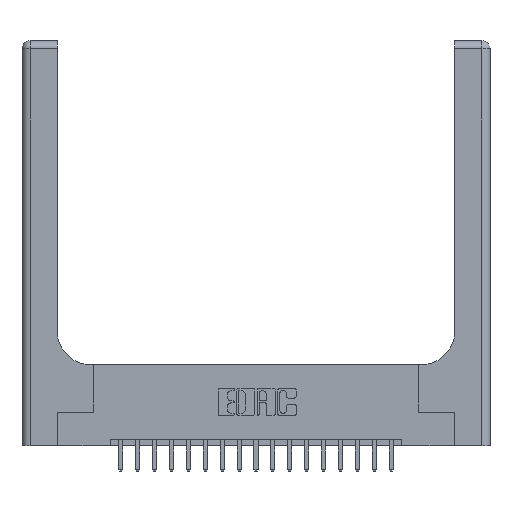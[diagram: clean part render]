
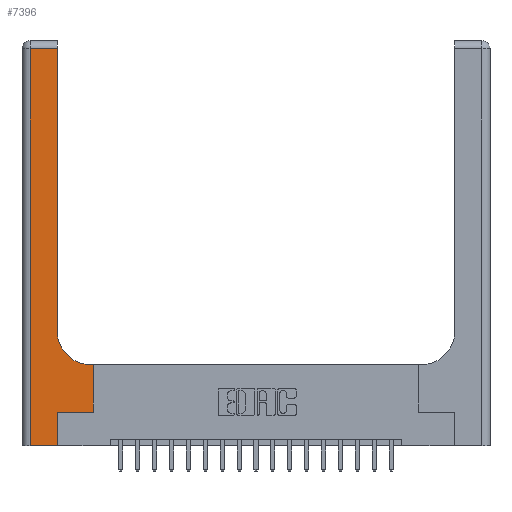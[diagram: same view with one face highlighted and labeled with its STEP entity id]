
A CAD part, top view. The second image highlights one B-rep face of the part: STEP entity #7396.
In plain terms, the highlighted planar face has unit normal (0, 0, 1).
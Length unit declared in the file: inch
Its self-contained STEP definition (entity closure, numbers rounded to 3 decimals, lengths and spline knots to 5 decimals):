
#52 = CARTESIAN_POINT ( 'NONE',  ( 0.26, 0.6, 0.37 ) ) ;
#112 = LINE ( 'NONE', #11116, #958 ) ;
#550 = CARTESIAN_POINT ( 'NONE',  ( 0.265, 0., 0.37 ) ) ;
#718 = CARTESIAN_POINT ( 'NONE',  ( 0.26, 2.94, 0.37 ) ) ;
#727 = CARTESIAN_POINT ( 'NONE',  ( 0., 0., 0.37 ) ) ;
#887 = ORIENTED_EDGE ( 'NONE', *, *, #5581, .T. ) ;
#958 = VECTOR ( 'NONE', #15806, 39.37008 ) ;
#1200 = LINE ( 'NONE', #727, #9588 ) ;
#1268 = EDGE_CURVE ( 'NONE', #19633, #1485, #16628, .T. ) ;
#1485 = VERTEX_POINT ( 'NONE', #2254 ) ;
#1619 = DIRECTION ( 'NONE',  ( -1., 0., 0. ) ) ;
#1894 = LINE ( 'NONE', #550, #2456 ) ;
#2235 = ORIENTED_EDGE ( 'NONE', *, *, #10881, .T. ) ;
#2254 = CARTESIAN_POINT ( 'NONE',  ( 0.06, 0., 0.37 ) ) ;
#2456 = VECTOR ( 'NONE', #17449, 39.37008 ) ;
#3403 = CARTESIAN_POINT ( 'NONE',  ( 0.265, 0.25, 0.37 ) ) ;
#3526 = VERTEX_POINT ( 'NONE', #4271 ) ;
#3614 = EDGE_CURVE ( 'NONE', #3526, #9872, #14115, .T. ) ;
#4226 = LINE ( 'NONE', #13772, #12684 ) ;
#4271 = CARTESIAN_POINT ( 'NONE',  ( 0.528, 0.6, 0.37 ) ) ;
#4289 = CARTESIAN_POINT ( 'NONE',  ( 0.06, 2.94, 0.37 ) ) ;
#4811 = AXIS2_PLACEMENT_3D ( 'NONE', #14265, #14073, #17016 ) ;
#5474 = DIRECTION ( 'NONE',  ( 0., -1., 0. ) ) ;
#5581 = EDGE_CURVE ( 'NONE', #6581, #9109, #112, .T. ) ;
#5914 = PLANE ( 'NONE',  #20081 ) ;
#5966 = DIRECTION ( 'NONE',  ( 1., 0., 0. ) ) ;
#6322 = DIRECTION ( 'NONE',  ( -1., 0., 0. ) ) ;
#6462 = ORIENTED_EDGE ( 'NONE', *, *, #18811, .T. ) ;
#6581 = VERTEX_POINT ( 'NONE', #7787 ) ;
#6842 = LINE ( 'NONE', #7458, #16123 ) ;
#7328 = ORIENTED_EDGE ( 'NONE', *, *, #3614, .T. ) ;
#7396 = ADVANCED_FACE ( 'NONE', ( #17382 ), #5914, .F. ) ;
#7412 = ORIENTED_EDGE ( 'NONE', *, *, #16473, .T. ) ;
#7458 = CARTESIAN_POINT ( 'NONE',  ( 0.265, 0.25, 0.37 ) ) ;
#7520 = ORIENTED_EDGE ( 'NONE', *, *, #16606, .T. ) ;
#7787 = CARTESIAN_POINT ( 'NONE',  ( 0.26, 0.85, 0.37 ) ) ;
#7793 = EDGE_CURVE ( 'NONE', #9057, #3526, #8575, .T. ) ;
#7808 = CARTESIAN_POINT ( 'NONE',  ( 0.51, 0.6, 0.37 ) ) ;
#8575 = LINE ( 'NONE', #11718, #14574 ) ;
#9057 = VERTEX_POINT ( 'NONE', #17623 ) ;
#9109 = VERTEX_POINT ( 'NONE', #718 ) ;
#9375 = CARTESIAN_POINT ( 'NONE',  ( 0.265, 0., 0.37 ) ) ;
#9588 = VECTOR ( 'NONE', #5966, 39.37008 ) ;
#9872 = VERTEX_POINT ( 'NONE', #7808 ) ;
#10029 = VECTOR ( 'NONE', #5474, 39.37008 ) ;
#10498 = DIRECTION ( 'NONE',  ( 0., 1., 0. ) ) ;
#10881 = EDGE_CURVE ( 'NONE', #1485, #17893, #1200, .T. ) ;
#11116 = CARTESIAN_POINT ( 'NONE',  ( 0.26, 3., 0.37 ) ) ;
#11326 = ORIENTED_EDGE ( 'NONE', *, *, #1268, .T. ) ;
#11406 = EDGE_LOOP ( 'NONE', ( #887, #7412, #11326, #2235, #6462, #12799, #16649, #7328, #7520 ) ) ;
#11561 = EDGE_CURVE ( 'NONE', #19064, #9057, #6842, .T. ) ;
#11718 = CARTESIAN_POINT ( 'NONE',  ( 0.528, 0.25, 0.37 ) ) ;
#12050 = DIRECTION ( 'NONE',  ( 1., 0., 0. ) ) ;
#12684 = VECTOR ( 'NONE', #16711, 39.37008 ) ;
#12799 = ORIENTED_EDGE ( 'NONE', *, *, #11561, .T. ) ;
#13772 = CARTESIAN_POINT ( 'NONE',  ( 0., 2.94, 0.37 ) ) ;
#13783 = DIRECTION ( 'NONE',  ( 0., 0., -1. ) ) ;
#14073 = DIRECTION ( 'NONE',  ( 0., 0., -1. ) ) ;
#14115 = LINE ( 'NONE', #52, #18869 ) ;
#14265 = CARTESIAN_POINT ( 'NONE',  ( 0.51, 0.85, 0.37 ) ) ;
#14574 = VECTOR ( 'NONE', #10498, 39.37008 ) ;
#15806 = DIRECTION ( 'NONE',  ( 0., 1., 0. ) ) ;
#16123 = VECTOR ( 'NONE', #12050, 39.37008 ) ;
#16473 = EDGE_CURVE ( 'NONE', #9109, #19633, #4226, .T. ) ;
#16606 = EDGE_CURVE ( 'NONE', #9872, #6581, #17527, .T. ) ;
#16628 = LINE ( 'NONE', #19457, #10029 ) ;
#16649 = ORIENTED_EDGE ( 'NONE', *, *, #7793, .T. ) ;
#16711 = DIRECTION ( 'NONE',  ( -1., 0., 0. ) ) ;
#17016 = DIRECTION ( 'NONE',  ( 1., 0., 0. ) ) ;
#17382 = FACE_OUTER_BOUND ( 'NONE', #11406, .T. ) ;
#17449 = DIRECTION ( 'NONE',  ( 0., 1., 0. ) ) ;
#17527 = CIRCLE ( 'NONE', #4811, 0.25 ) ;
#17623 = CARTESIAN_POINT ( 'NONE',  ( 0.528, 0.25, 0.37 ) ) ;
#17893 = VERTEX_POINT ( 'NONE', #9375 ) ;
#18811 = EDGE_CURVE ( 'NONE', #17893, #19064, #1894, .T. ) ;
#18818 = CARTESIAN_POINT ( 'NONE',  ( 0., 3., 0.37 ) ) ;
#18869 = VECTOR ( 'NONE', #6322, 39.37008 ) ;
#19064 = VERTEX_POINT ( 'NONE', #3403 ) ;
#19457 = CARTESIAN_POINT ( 'NONE',  ( 0.06, 3., 0.37 ) ) ;
#19633 = VERTEX_POINT ( 'NONE', #4289 ) ;
#20081 = AXIS2_PLACEMENT_3D ( 'NONE', #18818, #13783, #1619 ) ;
